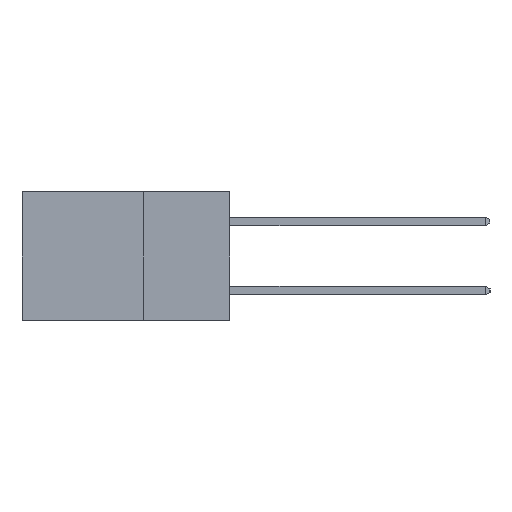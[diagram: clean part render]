
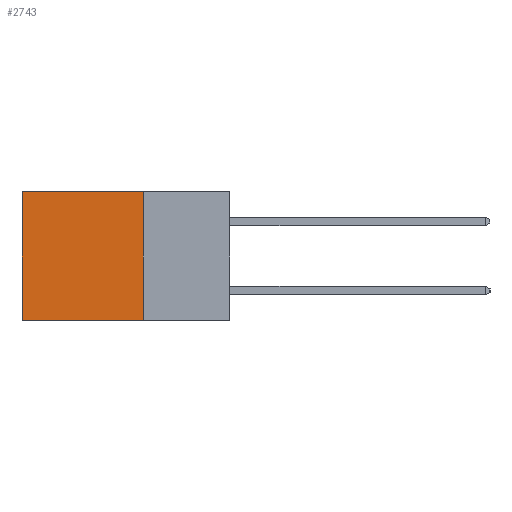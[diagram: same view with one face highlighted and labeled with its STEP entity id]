
A CAD part, left-side view. The second image highlights one B-rep face of the part: STEP entity #2743.
In plain terms, the highlighted planar face has unit normal (-1, 0, 0).
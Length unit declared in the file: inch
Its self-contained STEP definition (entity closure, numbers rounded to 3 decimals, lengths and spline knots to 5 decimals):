
#360 = VERTEX_POINT ( 'NONE', #10709 ) ;
#429 = VECTOR ( 'NONE', #2259, 39.37008 ) ;
#901 = VERTEX_POINT ( 'NONE', #9511 ) ;
#1053 = LINE ( 'NONE', #1435, #9862 ) ;
#1198 = EDGE_CURVE ( 'NONE', #4428, #360, #7678, .T. ) ;
#1214 = FACE_OUTER_BOUND ( 'NONE', #2932, .T. ) ;
#1435 = CARTESIAN_POINT ( 'NONE',  ( 0.2615, 0.6, -0.37 ) ) ;
#1478 = VECTOR ( 'NONE', #5596, 39.37008 ) ;
#2080 = EDGE_CURVE ( 'NONE', #360, #7253, #3089, .T. ) ;
#2112 = CARTESIAN_POINT ( 'NONE',  ( 0.2615, 0.25, 0. ) ) ;
#2259 = DIRECTION ( 'NONE',  ( 0., 0., -1. ) ) ;
#2743 = ADVANCED_FACE ( 'NONE', ( #1214 ), #5194, .F. ) ;
#2932 = EDGE_LOOP ( 'NONE', ( #6552, #6650, #6722, #6933 ) ) ;
#3089 = LINE ( 'NONE', #5786, #7417 ) ;
#3092 = EDGE_CURVE ( 'NONE', #4428, #901, #8381, .T. ) ;
#4428 = VERTEX_POINT ( 'NONE', #2112 ) ;
#4863 = CARTESIAN_POINT ( 'NONE',  ( 0.2615, 0.25, -0.37 ) ) ;
#4990 = AXIS2_PLACEMENT_3D ( 'NONE', #4863, #5046, #5033 ) ;
#5033 = DIRECTION ( 'NONE',  ( 0., 0., -1. ) ) ;
#5046 = DIRECTION ( 'NONE',  ( 1., 0., 0. ) ) ;
#5194 = PLANE ( 'NONE',  #4990 ) ;
#5596 = DIRECTION ( 'NONE',  ( 0., 1., 0. ) ) ;
#5786 = CARTESIAN_POINT ( 'NONE',  ( 0.2615, 0.25, -0.37 ) ) ;
#5946 = DIRECTION ( 'NONE',  ( 0., 1., 0. ) ) ;
#5954 = CARTESIAN_POINT ( 'NONE',  ( 0.2615, 0.6, -0.37 ) ) ;
#5984 = CARTESIAN_POINT ( 'NONE',  ( 0.2615, 0.25, 0. ) ) ;
#6552 = ORIENTED_EDGE ( 'NONE', *, *, #10351, .T. ) ;
#6650 = ORIENTED_EDGE ( 'NONE', *, *, #2080, .F. ) ;
#6722 = ORIENTED_EDGE ( 'NONE', *, *, #1198, .F. ) ;
#6933 = ORIENTED_EDGE ( 'NONE', *, *, #3092, .T. ) ;
#7253 = VERTEX_POINT ( 'NONE', #5954 ) ;
#7417 = VECTOR ( 'NONE', #5946, 39.37008 ) ;
#7678 = LINE ( 'NONE', #7758, #429 ) ;
#7758 = CARTESIAN_POINT ( 'NONE',  ( 0.2615, 0.25, -0.37 ) ) ;
#8354 = DIRECTION ( 'NONE',  ( 0., 0., -1. ) ) ;
#8381 = LINE ( 'NONE', #5984, #1478 ) ;
#9511 = CARTESIAN_POINT ( 'NONE',  ( 0.2615, 0.6, 0. ) ) ;
#9862 = VECTOR ( 'NONE', #8354, 39.37008 ) ;
#10351 = EDGE_CURVE ( 'NONE', #901, #7253, #1053, .T. ) ;
#10709 = CARTESIAN_POINT ( 'NONE',  ( 0.2615, 0.25, -0.37 ) ) ;
